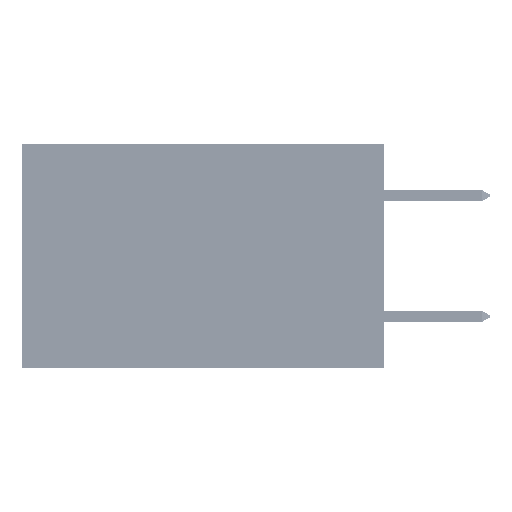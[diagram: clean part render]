
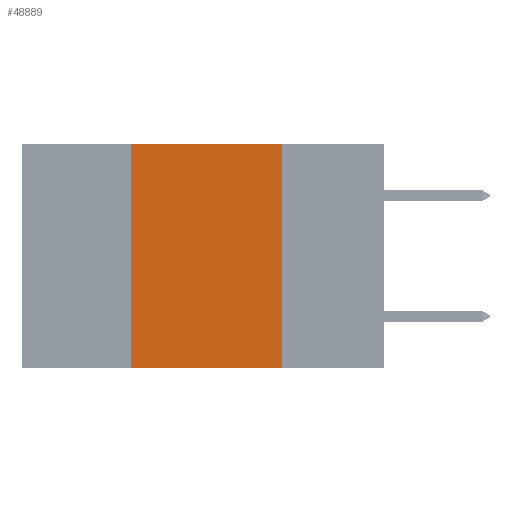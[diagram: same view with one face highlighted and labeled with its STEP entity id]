
A CAD part, left-side view. The second image highlights one B-rep face of the part: STEP entity #48889.
In plain terms, the highlighted planar face has unit normal (-1, 0, 0).
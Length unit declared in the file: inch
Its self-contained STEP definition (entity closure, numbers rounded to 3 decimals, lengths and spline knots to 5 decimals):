
#327 = CARTESIAN_POINT ( 'NONE',  ( 0., 0.6, 0. ) ) ;
#2304 = CARTESIAN_POINT ( 'NONE',  ( 0., 0.6, -0.37 ) ) ;
#3375 = DIRECTION ( 'NONE',  ( 0., 0., 1. ) ) ;
#5046 = VERTEX_POINT ( 'NONE', #27776 ) ;
#6461 = VERTEX_POINT ( 'NONE', #45388 ) ;
#8065 = DIRECTION ( 'NONE',  ( 0., -1., 0. ) ) ;
#8285 = VECTOR ( 'NONE', #8065, 39.37008 ) ;
#8391 = ORIENTED_EDGE ( 'NONE', *, *, #28690, .T. ) ;
#8816 = VECTOR ( 'NONE', #3375, 39.37008 ) ;
#12653 = CARTESIAN_POINT ( 'NONE',  ( 0., 0.42, 0. ) ) ;
#14029 = ORIENTED_EDGE ( 'NONE', *, *, #37680, .F. ) ;
#15906 = DIRECTION ( 'NONE',  ( 1., 0., 0. ) ) ;
#16522 = VECTOR ( 'NONE', #36426, 39.37008 ) ;
#17920 = ORIENTED_EDGE ( 'NONE', *, *, #37109, .F. ) ;
#19042 = LINE ( 'NONE', #20066, #8285 ) ;
#20066 = CARTESIAN_POINT ( 'NONE',  ( 0., 0.6, 0. ) ) ;
#20165 = LINE ( 'NONE', #33809, #8816 ) ;
#20706 = VERTEX_POINT ( 'NONE', #12653 ) ;
#21086 = CARTESIAN_POINT ( 'NONE',  ( 0., 0.17, 0. ) ) ;
#23262 = PLANE ( 'NONE',  #27383 ) ;
#23654 = VECTOR ( 'NONE', #29044, 39.37008 ) ;
#25153 = FACE_OUTER_BOUND ( 'NONE', #28950, .T. ) ;
#27383 = AXIS2_PLACEMENT_3D ( 'NONE', #327, #15906, #46202 ) ;
#27776 = CARTESIAN_POINT ( 'NONE',  ( 0., 0.17, -0.37 ) ) ;
#27913 = LINE ( 'NONE', #21086, #16522 ) ;
#28690 = EDGE_CURVE ( 'NONE', #6461, #5046, #36164, .T. ) ;
#28950 = EDGE_LOOP ( 'NONE', ( #14029, #47038, #17920, #8391 ) ) ;
#29044 = DIRECTION ( 'NONE',  ( 0., -1., 0. ) ) ;
#33182 = CARTESIAN_POINT ( 'NONE',  ( 0., 0.17, 0. ) ) ;
#33809 = CARTESIAN_POINT ( 'NONE',  ( 0., 0.42, 0. ) ) ;
#36164 = LINE ( 'NONE', #2304, #23654 ) ;
#36228 = EDGE_CURVE ( 'NONE', #20706, #46761, #19042, .T. ) ;
#36426 = DIRECTION ( 'NONE',  ( 0., 0., -1. ) ) ;
#37109 = EDGE_CURVE ( 'NONE', #6461, #20706, #20165, .T. ) ;
#37680 = EDGE_CURVE ( 'NONE', #46761, #5046, #27913, .T. ) ;
#45388 = CARTESIAN_POINT ( 'NONE',  ( 0., 0.42, -0.37 ) ) ;
#46202 = DIRECTION ( 'NONE',  ( 0., 0., -1. ) ) ;
#46761 = VERTEX_POINT ( 'NONE', #33182 ) ;
#47038 = ORIENTED_EDGE ( 'NONE', *, *, #36228, .F. ) ;
#48889 = ADVANCED_FACE ( 'NONE', ( #25153 ), #23262, .F. ) ;
